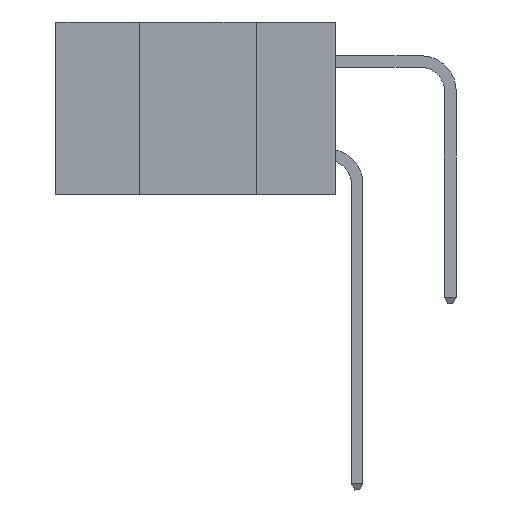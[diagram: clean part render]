
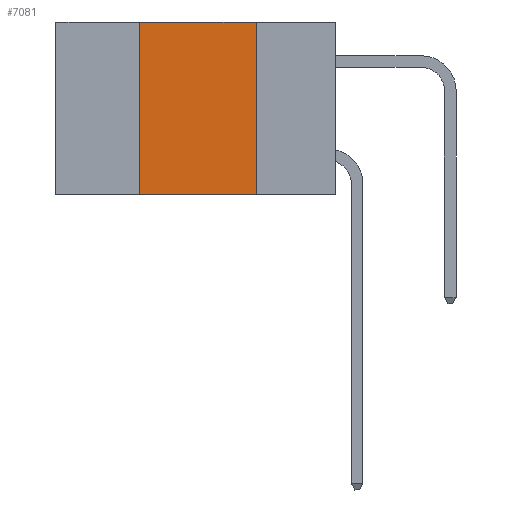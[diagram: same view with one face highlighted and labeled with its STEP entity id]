
A CAD part, left-side view. The second image highlights one B-rep face of the part: STEP entity #7081.
In plain terms, the highlighted planar face has unit normal (-1, 0, 0).
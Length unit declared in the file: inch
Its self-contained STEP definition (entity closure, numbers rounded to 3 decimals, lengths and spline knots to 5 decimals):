
#1380 = VECTOR ( 'NONE', #17878, 39.37008 ) ;
#3349 = LINE ( 'NONE', #25061, #17338 ) ;
#3481 = EDGE_CURVE ( 'NONE', #6899, #7876, #3349, .T. ) ;
#4345 = EDGE_CURVE ( 'NONE', #23875, #12149, #11891, .T. ) ;
#6294 = VECTOR ( 'NONE', #24439, 39.37008 ) ;
#6899 = VERTEX_POINT ( 'NONE', #23516 ) ;
#7081 = ADVANCED_FACE ( 'NONE', ( #20965 ), #7618, .F. ) ;
#7618 = PLANE ( 'NONE',  #29793 ) ;
#7876 = VERTEX_POINT ( 'NONE', #27796 ) ;
#9577 = CARTESIAN_POINT ( 'NONE',  ( 0., 0.17, 0. ) ) ;
#9930 = CARTESIAN_POINT ( 'NONE',  ( 0., 0.6, 0. ) ) ;
#10127 = DIRECTION ( 'NONE',  ( 1., 0., 0. ) ) ;
#10209 = DIRECTION ( 'NONE',  ( 0., 0., 1. ) ) ;
#10914 = ORIENTED_EDGE ( 'NONE', *, *, #4345, .F. ) ;
#11347 = LINE ( 'NONE', #26426, #18679 ) ;
#11555 = DIRECTION ( 'NONE',  ( 0., -1., 0. ) ) ;
#11891 = LINE ( 'NONE', #25176, #1380 ) ;
#12149 = VERTEX_POINT ( 'NONE', #30831 ) ;
#13912 = EDGE_LOOP ( 'NONE', ( #10914, #17289, #21661, #26912 ) ) ;
#17289 = ORIENTED_EDGE ( 'NONE', *, *, #18009, .F. ) ;
#17338 = VECTOR ( 'NONE', #10209, 39.37008 ) ;
#17878 = DIRECTION ( 'NONE',  ( 0., 0., -1. ) ) ;
#18009 = EDGE_CURVE ( 'NONE', #7876, #23875, #29655, .T. ) ;
#18463 = EDGE_CURVE ( 'NONE', #6899, #12149, #11347, .T. ) ;
#18679 = VECTOR ( 'NONE', #11555, 39.37008 ) ;
#20965 = FACE_OUTER_BOUND ( 'NONE', #13912, .T. ) ;
#21661 = ORIENTED_EDGE ( 'NONE', *, *, #3481, .F. ) ;
#23227 = CARTESIAN_POINT ( 'NONE',  ( 0., 0.6, 0. ) ) ;
#23516 = CARTESIAN_POINT ( 'NONE',  ( 0., 0.42, -0.37 ) ) ;
#23875 = VERTEX_POINT ( 'NONE', #9577 ) ;
#24439 = DIRECTION ( 'NONE',  ( 0., -1., 0. ) ) ;
#25061 = CARTESIAN_POINT ( 'NONE',  ( 0., 0.42, 0. ) ) ;
#25176 = CARTESIAN_POINT ( 'NONE',  ( 0., 0.17, 0. ) ) ;
#26426 = CARTESIAN_POINT ( 'NONE',  ( 0., 0.6, -0.37 ) ) ;
#26912 = ORIENTED_EDGE ( 'NONE', *, *, #18463, .T. ) ;
#27595 = DIRECTION ( 'NONE',  ( 0., 0., -1. ) ) ;
#27796 = CARTESIAN_POINT ( 'NONE',  ( 0., 0.42, 0. ) ) ;
#29655 = LINE ( 'NONE', #23227, #6294 ) ;
#29793 = AXIS2_PLACEMENT_3D ( 'NONE', #9930, #10127, #27595 ) ;
#30831 = CARTESIAN_POINT ( 'NONE',  ( 0., 0.17, -0.37 ) ) ;
